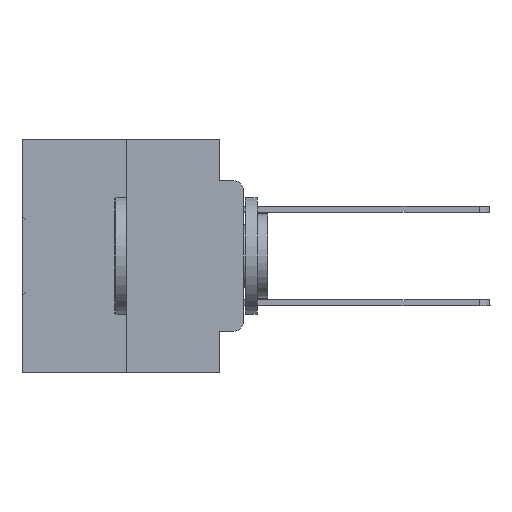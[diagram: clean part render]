
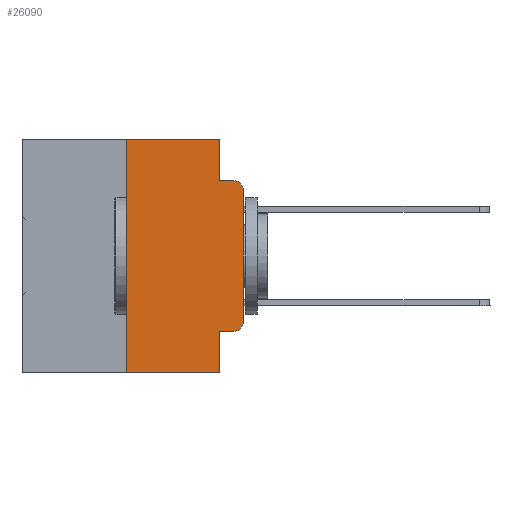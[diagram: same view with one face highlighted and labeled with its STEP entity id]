
A CAD part, left-side view. The second image highlights one B-rep face of the part: STEP entity #26090.
In plain terms, the highlighted planar face has unit normal (-1, 0, 0).
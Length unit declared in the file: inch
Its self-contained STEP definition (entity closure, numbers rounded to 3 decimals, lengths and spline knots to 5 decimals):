
#242 = ORIENTED_EDGE ( 'NONE', *, *, #30108, .F. ) ;
#483 = CARTESIAN_POINT ( 'NONE',  ( 0., 0.02, -0.3915 ) ) ;
#1063 = CARTESIAN_POINT ( 'NONE',  ( 0., 0.051, 0. ) ) ;
#2003 = CARTESIAN_POINT ( 'NONE',  ( 0., 0.051, -0.4115 ) ) ;
#2359 = DIRECTION ( 'NONE',  ( 0., 0., -1. ) ) ;
#2600 = CARTESIAN_POINT ( 'NONE',  ( 0., 0.25, 0. ) ) ;
#2659 = EDGE_LOOP ( 'NONE', ( #15393, #17518, #11045, #242, #24244, #4725, #8687, #8927, #21284, #7859 ) ) ;
#3098 = EDGE_CURVE ( 'NONE', #7403, #35705, #7005, .T. ) ;
#3184 = DIRECTION ( 'NONE',  ( 0., -1., 0. ) ) ;
#3414 = DIRECTION ( 'NONE',  ( -1., 0., 0. ) ) ;
#4257 = DIRECTION ( 'NONE',  ( 0., 0., 1. ) ) ;
#4725 = ORIENTED_EDGE ( 'NONE', *, *, #7439, .F. ) ;
#5798 = LINE ( 'NONE', #8177, #7904 ) ;
#5924 = LINE ( 'NONE', #23108, #24438 ) ;
#6659 = VERTEX_POINT ( 'NONE', #13682 ) ;
#6934 = CARTESIAN_POINT ( 'NONE',  ( 0., 0.02, -0.4115 ) ) ;
#7005 = LINE ( 'NONE', #26743, #29925 ) ;
#7403 = VERTEX_POINT ( 'NONE', #29453 ) ;
#7439 = EDGE_CURVE ( 'NONE', #8634, #14465, #32197, .T. ) ;
#7712 = CARTESIAN_POINT ( 'NONE',  ( 0., 0.051, -0.4115 ) ) ;
#7859 = ORIENTED_EDGE ( 'NONE', *, *, #20396, .T. ) ;
#7904 = VECTOR ( 'NONE', #27614, 39.37008 ) ;
#8177 = CARTESIAN_POINT ( 'NONE',  ( 0., 0.051, 0. ) ) ;
#8634 = VERTEX_POINT ( 'NONE', #25390 ) ;
#8687 = ORIENTED_EDGE ( 'NONE', *, *, #14056, .T. ) ;
#8927 = ORIENTED_EDGE ( 'NONE', *, *, #18906, .F. ) ;
#9131 = VECTOR ( 'NONE', #32762, 39.37008 ) ;
#9440 = DIRECTION ( 'NONE',  ( 0., 0., -1. ) ) ;
#9617 = LINE ( 'NONE', #32073, #21201 ) ;
#11045 = ORIENTED_EDGE ( 'NONE', *, *, #33190, .F. ) ;
#12912 = CARTESIAN_POINT ( 'NONE',  ( 0., 0.473, -0.5 ) ) ;
#13201 = EDGE_CURVE ( 'NONE', #20978, #35528, #15790, .T. ) ;
#13211 = CARTESIAN_POINT ( 'NONE',  ( 0., 0.051, -0.5 ) ) ;
#13342 = FACE_OUTER_BOUND ( 'NONE', #2659, .T. ) ;
#13682 = CARTESIAN_POINT ( 'NONE',  ( 0., 0.051, 0. ) ) ;
#14056 = EDGE_CURVE ( 'NONE', #8634, #29148, #15662, .T. ) ;
#14465 = VERTEX_POINT ( 'NONE', #2600 ) ;
#14847 = AXIS2_PLACEMENT_3D ( 'NONE', #29938, #32155, #2359 ) ;
#15393 = ORIENTED_EDGE ( 'NONE', *, *, #3098, .T. ) ;
#15662 = LINE ( 'NONE', #12912, #25433 ) ;
#15790 = LINE ( 'NONE', #7712, #9131 ) ;
#16378 = VERTEX_POINT ( 'NONE', #35018 ) ;
#17518 = ORIENTED_EDGE ( 'NONE', *, *, #20481, .T. ) ;
#17624 = VERTEX_POINT ( 'NONE', #35376 ) ;
#18279 = CIRCLE ( 'NONE', #26449, 0.02 ) ;
#18906 = EDGE_CURVE ( 'NONE', #20978, #29148, #22994, .T. ) ;
#20396 = EDGE_CURVE ( 'NONE', #35528, #7403, #20630, .T. ) ;
#20481 = EDGE_CURVE ( 'NONE', #35705, #16378, #18279, .T. ) ;
#20549 = EDGE_CURVE ( 'NONE', #14465, #6659, #9617, .T. ) ;
#20630 = CIRCLE ( 'NONE', #34616, 0.02 ) ;
#20978 = VERTEX_POINT ( 'NONE', #2003 ) ;
#21201 = VECTOR ( 'NONE', #29500, 39.37008 ) ;
#21202 = PLANE ( 'NONE',  #14847 ) ;
#21284 = ORIENTED_EDGE ( 'NONE', *, *, #13201, .T. ) ;
#21797 = VECTOR ( 'NONE', #34124, 39.37008 ) ;
#22994 = LINE ( 'NONE', #1063, #21797 ) ;
#23108 = CARTESIAN_POINT ( 'NONE',  ( 0., 0.051, -0.0885 ) ) ;
#23238 = VECTOR ( 'NONE', #34760, 39.37008 ) ;
#23691 = CARTESIAN_POINT ( 'NONE',  ( 0., 0.02, -0.1085 ) ) ;
#23996 = CARTESIAN_POINT ( 'NONE',  ( 0., 0.25, 0. ) ) ;
#24219 = DIRECTION ( 'NONE',  ( 0., 0., -1. ) ) ;
#24244 = ORIENTED_EDGE ( 'NONE', *, *, #20549, .F. ) ;
#24438 = VECTOR ( 'NONE', #3184, 39.37008 ) ;
#25390 = CARTESIAN_POINT ( 'NONE',  ( 0., 0.25, -0.5 ) ) ;
#25433 = VECTOR ( 'NONE', #35171, 39.37008 ) ;
#26090 = ADVANCED_FACE ( 'NONE', ( #13342 ), #21202, .F. ) ;
#26449 = AXIS2_PLACEMENT_3D ( 'NONE', #23691, #32623, #24219 ) ;
#26743 = CARTESIAN_POINT ( 'NONE',  ( 0., 0., 0. ) ) ;
#27614 = DIRECTION ( 'NONE',  ( 0., 0., -1. ) ) ;
#29148 = VERTEX_POINT ( 'NONE', #13211 ) ;
#29453 = CARTESIAN_POINT ( 'NONE',  ( 0., 0., -0.3915 ) ) ;
#29500 = DIRECTION ( 'NONE',  ( 0., -1., 0. ) ) ;
#29925 = VECTOR ( 'NONE', #4257, 39.37008 ) ;
#29938 = CARTESIAN_POINT ( 'NONE',  ( 0., 0.473, 0. ) ) ;
#30108 = EDGE_CURVE ( 'NONE', #6659, #17624, #5798, .T. ) ;
#30293 = CARTESIAN_POINT ( 'NONE',  ( 0., 0., -0.1085 ) ) ;
#32073 = CARTESIAN_POINT ( 'NONE',  ( 0., 0.473, 0. ) ) ;
#32155 = DIRECTION ( 'NONE',  ( 1., 0., 0. ) ) ;
#32197 = LINE ( 'NONE', #23996, #23238 ) ;
#32623 = DIRECTION ( 'NONE',  ( -1., 0., 0. ) ) ;
#32762 = DIRECTION ( 'NONE',  ( 0., -1., 0. ) ) ;
#33190 = EDGE_CURVE ( 'NONE', #17624, #16378, #5924, .T. ) ;
#34124 = DIRECTION ( 'NONE',  ( 0., 0., -1. ) ) ;
#34616 = AXIS2_PLACEMENT_3D ( 'NONE', #483, #3414, #9440 ) ;
#34760 = DIRECTION ( 'NONE',  ( 0., 0., 1. ) ) ;
#35018 = CARTESIAN_POINT ( 'NONE',  ( 0., 0.02, -0.0885 ) ) ;
#35171 = DIRECTION ( 'NONE',  ( 0., -1., 0. ) ) ;
#35376 = CARTESIAN_POINT ( 'NONE',  ( 0., 0.051, -0.0885 ) ) ;
#35528 = VERTEX_POINT ( 'NONE', #6934 ) ;
#35705 = VERTEX_POINT ( 'NONE', #30293 ) ;
